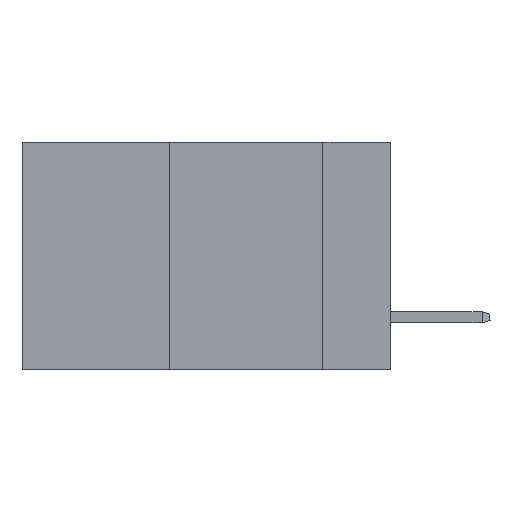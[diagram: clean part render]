
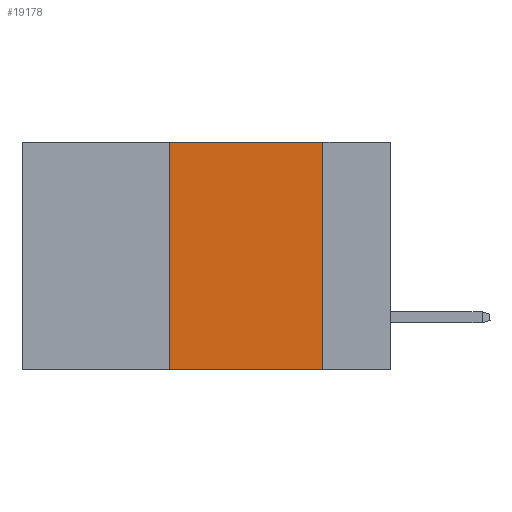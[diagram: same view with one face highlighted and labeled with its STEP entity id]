
A CAD part, left-side view. The second image highlights one B-rep face of the part: STEP entity #19178.
In plain terms, the highlighted planar face has unit normal (-1, 0, 0).
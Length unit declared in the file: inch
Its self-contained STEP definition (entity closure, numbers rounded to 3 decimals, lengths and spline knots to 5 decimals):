
#12 = VERTEX_POINT ( 'NONE', #35534 ) ;
#551 = FACE_OUTER_BOUND ( 'NONE', #30409, .T. ) ;
#855 = EDGE_CURVE ( 'NONE', #6855, #5053, #3003, .T. ) ;
#1353 = EDGE_CURVE ( 'NONE', #6855, #12, #15783, .T. ) ;
#3003 = LINE ( 'NONE', #33529, #36563 ) ;
#4204 = DIRECTION ( 'NONE',  ( 0., -1., 0. ) ) ;
#5053 = VERTEX_POINT ( 'NONE', #30850 ) ;
#5959 = EDGE_CURVE ( 'NONE', #6780, #5053, #13218, .T. ) ;
#6564 = VECTOR ( 'NONE', #19389, 39.37008 ) ;
#6780 = VERTEX_POINT ( 'NONE', #41548 ) ;
#6855 = VERTEX_POINT ( 'NONE', #8883 ) ;
#8883 = CARTESIAN_POINT ( 'NONE',  ( 0., 0.36, -0.37 ) ) ;
#11343 = DIRECTION ( 'NONE',  ( 1., 0., 0. ) ) ;
#13218 = LINE ( 'NONE', #32614, #6564 ) ;
#14715 = VECTOR ( 'NONE', #19900, 39.37008 ) ;
#15783 = LINE ( 'NONE', #23353, #14715 ) ;
#16554 = ORIENTED_EDGE ( 'NONE', *, *, #5959, .F. ) ;
#18471 = EDGE_CURVE ( 'NONE', #12, #6780, #30126, .T. ) ;
#19178 = ADVANCED_FACE ( 'NONE', ( #551 ), #37756, .F. ) ;
#19389 = DIRECTION ( 'NONE',  ( 0., 0., -1. ) ) ;
#19900 = DIRECTION ( 'NONE',  ( 0., 0., 1. ) ) ;
#20468 = ORIENTED_EDGE ( 'NONE', *, *, #1353, .F. ) ;
#21217 = CARTESIAN_POINT ( 'NONE',  ( 0., 0.6, 0. ) ) ;
#22933 = ORIENTED_EDGE ( 'NONE', *, *, #18471, .F. ) ;
#23353 = CARTESIAN_POINT ( 'NONE',  ( 0., 0.36, 0. ) ) ;
#23390 = VECTOR ( 'NONE', #38099, 39.37008 ) ;
#26678 = ORIENTED_EDGE ( 'NONE', *, *, #855, .T. ) ;
#28371 = CARTESIAN_POINT ( 'NONE',  ( 0., 0.6, 0. ) ) ;
#30126 = LINE ( 'NONE', #28371, #23390 ) ;
#30409 = EDGE_LOOP ( 'NONE', ( #16554, #22933, #20468, #26678 ) ) ;
#30850 = CARTESIAN_POINT ( 'NONE',  ( 0., 0.11, -0.37 ) ) ;
#30955 = AXIS2_PLACEMENT_3D ( 'NONE', #21217, #11343, #34414 ) ;
#32614 = CARTESIAN_POINT ( 'NONE',  ( 0., 0.11, 0. ) ) ;
#33529 = CARTESIAN_POINT ( 'NONE',  ( 0., 0.6, -0.37 ) ) ;
#34414 = DIRECTION ( 'NONE',  ( 0., 0., -1. ) ) ;
#35534 = CARTESIAN_POINT ( 'NONE',  ( 0., 0.36, 0. ) ) ;
#36563 = VECTOR ( 'NONE', #4204, 39.37008 ) ;
#37756 = PLANE ( 'NONE',  #30955 ) ;
#38099 = DIRECTION ( 'NONE',  ( 0., -1., 0. ) ) ;
#41548 = CARTESIAN_POINT ( 'NONE',  ( 0., 0.11, 0. ) ) ;
